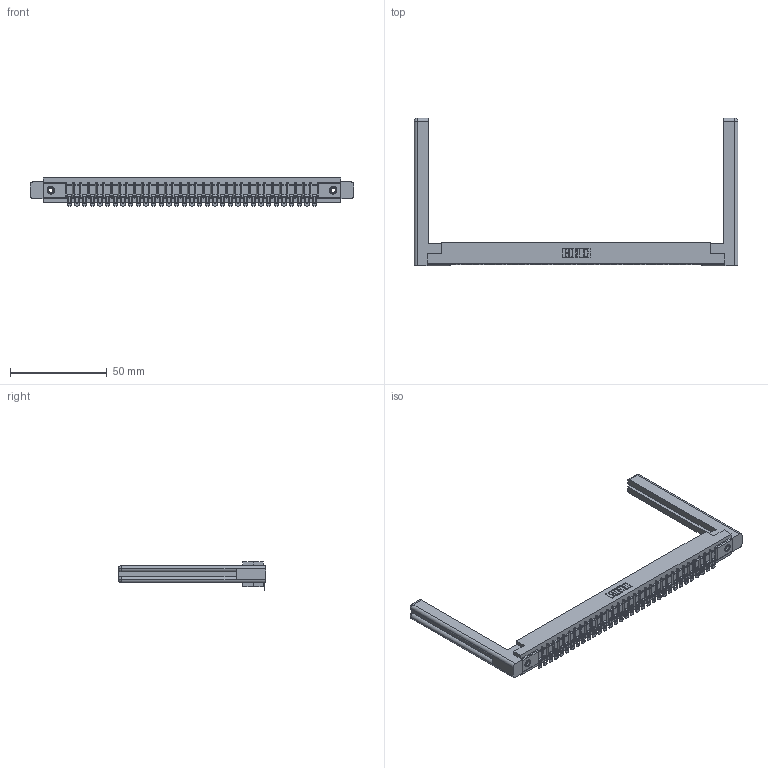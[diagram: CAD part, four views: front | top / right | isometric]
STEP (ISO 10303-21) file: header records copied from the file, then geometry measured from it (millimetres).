
FILE_DESCRIPTION (( 'STEP AP203' ), '1' );
FILE_NAME ('357-033-454-158.STEP', '2020-10-02T08:40:23', ( '' ), ( '' ), 'SwSTEP 2.0', 'SolidWorks 2020', '' );
FILE_SCHEMA (( 'CONFIG_CONTROL_DESIGN' ));
Length unit declared in the file: inch
Products named in the file (5): 345-250-001_345-250-001-102; 357-033-454-158; 307-290-002_554; 307-220-058; 307 Part_.156 Dia Mounting Holes
Assembly tree (38 placements, depth 2):
  357-033-454-158
    307 Part_.156 Dia Mounting Holes
    307-290-002_554  x33
    307-220-058  x2
    345-250-001_345-250-001-102  x2
Bounding box: 167.39 x 76.33 x 14.52 mm (x, y, z)
Volume: 24977.4 mm3; surface area: 27214.8 mm2
Topology: 38 solids, 38 shells, 2967 faces, 9026 edges, 5912 vertices
Faces by surface type: plane 1672, cylinder 1203, sphere 68, torus 12, cone 12
Entity records: 32998 total; most frequent: CARTESIAN_POINT 5573, ORIENTED_EDGE 5502, DIRECTION 5385, EDGE_CURVE 2751, VECTOR 2093, LINE 2093, VERTEX_POINT 1780, AXIS2_PLACEMENT_3D 1646
